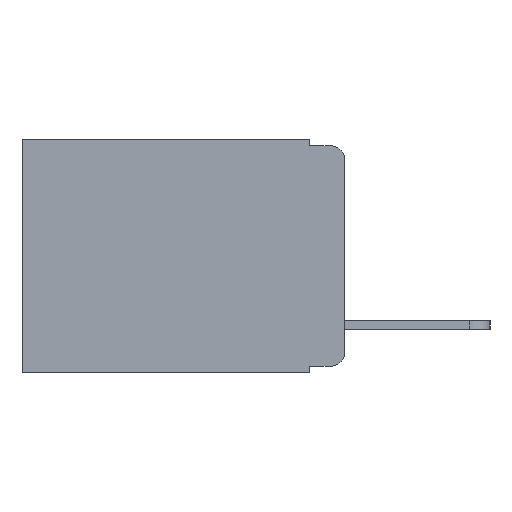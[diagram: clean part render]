
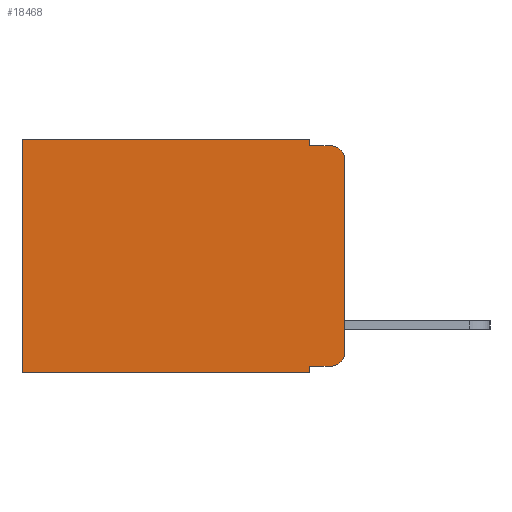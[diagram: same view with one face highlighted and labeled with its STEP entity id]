
A CAD part, left-side view. The second image highlights one B-rep face of the part: STEP entity #18468.
In plain terms, the highlighted planar face has unit normal (-1, 0, 0).
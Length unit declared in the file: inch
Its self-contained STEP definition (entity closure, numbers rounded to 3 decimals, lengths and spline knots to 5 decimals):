
#676 = DIRECTION ( 'NONE',  ( 0., 0., -1. ) ) ;
#1076 = VECTOR ( 'NONE', #8440, 39.37008 ) ;
#1401 = VERTEX_POINT ( 'NONE', #5390 ) ;
#1505 = VERTEX_POINT ( 'NONE', #21442 ) ;
#1742 = CARTESIAN_POINT ( 'NONE',  ( 0.298, 0., -0.03 ) ) ;
#1877 = CARTESIAN_POINT ( 'NONE',  ( 0.298, 0.051, 0. ) ) ;
#1967 = EDGE_CURVE ( 'NONE', #10211, #8613, #21027, .T. ) ;
#2335 = VECTOR ( 'NONE', #19379, 39.37008 ) ;
#2499 = CARTESIAN_POINT ( 'NONE',  ( 0.298, 0.051, 0. ) ) ;
#2636 = EDGE_LOOP ( 'NONE', ( #8346, #9518, #14751, #12496, #13646, #9510, #15688, #9676, #22360, #10775 ) ) ;
#3217 = FACE_OUTER_BOUND ( 'NONE', #2636, .T. ) ;
#3254 = CARTESIAN_POINT ( 'NONE',  ( 0.298, 0., 0. ) ) ;
#3454 = CARTESIAN_POINT ( 'NONE',  ( 0.298, 0.02, -0.313 ) ) ;
#3533 = EDGE_CURVE ( 'NONE', #10916, #1401, #18634, .T. ) ;
#3597 = DIRECTION ( 'NONE',  ( -1., 0., 0. ) ) ;
#3615 = VECTOR ( 'NONE', #12059, 39.37008 ) ;
#4154 = VECTOR ( 'NONE', #11765, 39.37008 ) ;
#4823 = VERTEX_POINT ( 'NONE', #1742 ) ;
#5153 = PLANE ( 'NONE',  #12945 ) ;
#5233 = EDGE_CURVE ( 'NONE', #8613, #15906, #14207, .T. ) ;
#5382 = DIRECTION ( 'NONE',  ( 0., 0., -1. ) ) ;
#5390 = CARTESIAN_POINT ( 'NONE',  ( 0.298, 0.02, -0.01 ) ) ;
#5405 = VERTEX_POINT ( 'NONE', #10880 ) ;
#5411 = LINE ( 'NONE', #3254, #1076 ) ;
#5504 = CARTESIAN_POINT ( 'NONE',  ( 0.298, 0.051, -0.333 ) ) ;
#8346 = ORIENTED_EDGE ( 'NONE', *, *, #15354, .F. ) ;
#8367 = VERTEX_POINT ( 'NONE', #1877 ) ;
#8440 = DIRECTION ( 'NONE',  ( 0., 1., 0. ) ) ;
#8492 = LINE ( 'NONE', #2499, #19443 ) ;
#8577 = CIRCLE ( 'NONE', #19984, 0.02 ) ;
#8613 = VERTEX_POINT ( 'NONE', #17972 ) ;
#8673 = LINE ( 'NONE', #18971, #8940 ) ;
#8940 = VECTOR ( 'NONE', #16405, 39.37008 ) ;
#8983 = EDGE_CURVE ( 'NONE', #13783, #5405, #8577, .T. ) ;
#8986 = EDGE_CURVE ( 'NONE', #4823, #1401, #15434, .T. ) ;
#9510 = ORIENTED_EDGE ( 'NONE', *, *, #15144, .T. ) ;
#9518 = ORIENTED_EDGE ( 'NONE', *, *, #8986, .T. ) ;
#9676 = ORIENTED_EDGE ( 'NONE', *, *, #1967, .F. ) ;
#10145 = LINE ( 'NONE', #18173, #12600 ) ;
#10211 = VERTEX_POINT ( 'NONE', #5504 ) ;
#10291 = CARTESIAN_POINT ( 'NONE',  ( 0.298, 0., -0.343 ) ) ;
#10433 = CARTESIAN_POINT ( 'NONE',  ( 0.298, 0.051, 0. ) ) ;
#10472 = DIRECTION ( 'NONE',  ( 1., 0., 0. ) ) ;
#10775 = ORIENTED_EDGE ( 'NONE', *, *, #8983, .T. ) ;
#10880 = CARTESIAN_POINT ( 'NONE',  ( 0.298, 0., -0.313 ) ) ;
#10916 = VERTEX_POINT ( 'NONE', #19915 ) ;
#11765 = DIRECTION ( 'NONE',  ( 0., 0., -1. ) ) ;
#12059 = DIRECTION ( 'NONE',  ( 0., 0., -1. ) ) ;
#12123 = CARTESIAN_POINT ( 'NONE',  ( 0.298, 0.473, -0.343 ) ) ;
#12496 = ORIENTED_EDGE ( 'NONE', *, *, #15046, .F. ) ;
#12600 = VECTOR ( 'NONE', #16186, 39.37008 ) ;
#12945 = AXIS2_PLACEMENT_3D ( 'NONE', #17370, #10472, #16038 ) ;
#13046 = EDGE_CURVE ( 'NONE', #10211, #13783, #8673, .T. ) ;
#13383 = EDGE_CURVE ( 'NONE', #8367, #1505, #5411, .T. ) ;
#13646 = ORIENTED_EDGE ( 'NONE', *, *, #13383, .T. ) ;
#13783 = VERTEX_POINT ( 'NONE', #16366 ) ;
#14207 = LINE ( 'NONE', #10291, #18303 ) ;
#14751 = ORIENTED_EDGE ( 'NONE', *, *, #3533, .F. ) ;
#15046 = EDGE_CURVE ( 'NONE', #8367, #10916, #8492, .T. ) ;
#15144 = EDGE_CURVE ( 'NONE', #1505, #15906, #10145, .T. ) ;
#15354 = EDGE_CURVE ( 'NONE', #4823, #5405, #17512, .T. ) ;
#15434 = CIRCLE ( 'NONE', #16784, 0.02 ) ;
#15573 = DIRECTION ( 'NONE',  ( 0., 1., 0. ) ) ;
#15617 = DIRECTION ( 'NONE',  ( -1., 0., 0. ) ) ;
#15688 = ORIENTED_EDGE ( 'NONE', *, *, #5233, .F. ) ;
#15906 = VERTEX_POINT ( 'NONE', #12123 ) ;
#16038 = DIRECTION ( 'NONE',  ( 0., 0., -1. ) ) ;
#16186 = DIRECTION ( 'NONE',  ( 0., 0., -1. ) ) ;
#16366 = CARTESIAN_POINT ( 'NONE',  ( 0.298, 0.02, -0.333 ) ) ;
#16405 = DIRECTION ( 'NONE',  ( 0., -1., 0. ) ) ;
#16784 = AXIS2_PLACEMENT_3D ( 'NONE', #21083, #3597, #5382 ) ;
#17370 = CARTESIAN_POINT ( 'NONE',  ( 0.298, 0., 0. ) ) ;
#17512 = LINE ( 'NONE', #18941, #4154 ) ;
#17972 = CARTESIAN_POINT ( 'NONE',  ( 0.298, 0.051, -0.343 ) ) ;
#18173 = CARTESIAN_POINT ( 'NONE',  ( 0.298, 0.473, 0. ) ) ;
#18303 = VECTOR ( 'NONE', #15573, 39.37008 ) ;
#18468 = ADVANCED_FACE ( 'NONE', ( #3217 ), #5153, .F. ) ;
#18634 = LINE ( 'NONE', #19457, #2335 ) ;
#18941 = CARTESIAN_POINT ( 'NONE',  ( 0.298, 0., 0. ) ) ;
#18971 = CARTESIAN_POINT ( 'NONE',  ( 0.298, 0.051, -0.333 ) ) ;
#19283 = DIRECTION ( 'NONE',  ( 0., 0., -1. ) ) ;
#19379 = DIRECTION ( 'NONE',  ( 0., -1., 0. ) ) ;
#19443 = VECTOR ( 'NONE', #676, 39.37008 ) ;
#19457 = CARTESIAN_POINT ( 'NONE',  ( 0.298, 0.051, -0.01 ) ) ;
#19915 = CARTESIAN_POINT ( 'NONE',  ( 0.298, 0.051, -0.01 ) ) ;
#19984 = AXIS2_PLACEMENT_3D ( 'NONE', #3454, #15617, #19283 ) ;
#21027 = LINE ( 'NONE', #10433, #3615 ) ;
#21083 = CARTESIAN_POINT ( 'NONE',  ( 0.298, 0.02, -0.03 ) ) ;
#21442 = CARTESIAN_POINT ( 'NONE',  ( 0.298, 0.473, 0. ) ) ;
#22360 = ORIENTED_EDGE ( 'NONE', *, *, #13046, .T. ) ;
